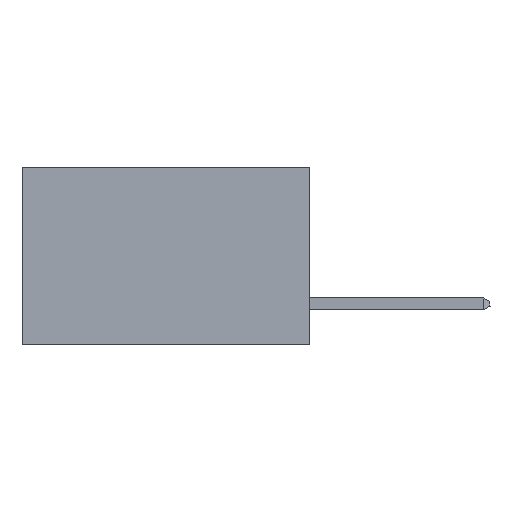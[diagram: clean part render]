
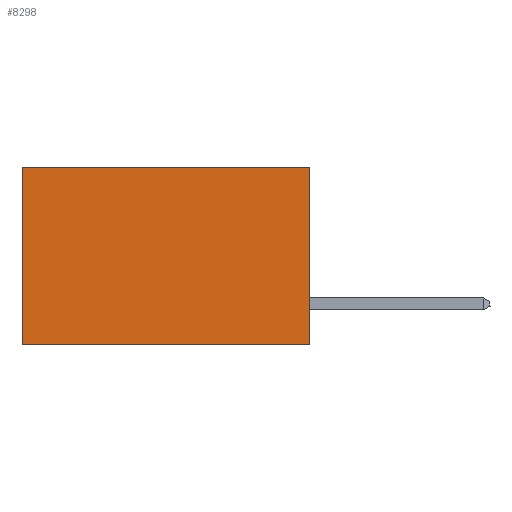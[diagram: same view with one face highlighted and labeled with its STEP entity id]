
A CAD part, left-side view. The second image highlights one B-rep face of the part: STEP entity #8298.
In plain terms, the highlighted planar face has unit normal (-1, 0, 0).
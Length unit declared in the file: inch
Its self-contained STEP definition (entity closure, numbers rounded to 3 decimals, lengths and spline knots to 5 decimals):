
#2330 = EDGE_CURVE ( 'NONE', #5590, #45355, #39319, .T. ) ;
#2902 = VECTOR ( 'NONE', #12301, 39.37008 ) ;
#4670 = CARTESIAN_POINT ( 'NONE',  ( 0.2875, 0., 0. ) ) ;
#5590 = VERTEX_POINT ( 'NONE', #4670 ) ;
#5637 = EDGE_CURVE ( 'NONE', #5590, #42489, #44893, .T. ) ;
#8045 = ORIENTED_EDGE ( 'NONE', *, *, #22477, .T. ) ;
#8128 = CARTESIAN_POINT ( 'NONE',  ( 0.2875, 0.6, 0. ) ) ;
#8298 = ADVANCED_FACE ( 'NONE', ( #40250 ), #26927, .F. ) ;
#8915 = LINE ( 'NONE', #32776, #2902 ) ;
#9253 = DIRECTION ( 'NONE',  ( 0., 0., -1. ) ) ;
#12110 = VECTOR ( 'NONE', #12383, 39.37008 ) ;
#12301 = DIRECTION ( 'NONE',  ( 0., 1., 0. ) ) ;
#12383 = DIRECTION ( 'NONE',  ( 0., 0., -1. ) ) ;
#12662 = CARTESIAN_POINT ( 'NONE',  ( 0.2875, 0., 0. ) ) ;
#14889 = CARTESIAN_POINT ( 'NONE',  ( 0.2875, 0.6, -0.37 ) ) ;
#21448 = LINE ( 'NONE', #8128, #12110 ) ;
#22477 = EDGE_CURVE ( 'NONE', #42489, #28965, #21448, .T. ) ;
#24565 = CARTESIAN_POINT ( 'NONE',  ( 0.2875, 0., 0. ) ) ;
#25160 = EDGE_LOOP ( 'NONE', ( #8045, #36801, #32295, #39297 ) ) ;
#25225 = CARTESIAN_POINT ( 'NONE',  ( 0.2875, 0., -0.37 ) ) ;
#26927 = PLANE ( 'NONE',  #27467 ) ;
#27467 = AXIS2_PLACEMENT_3D ( 'NONE', #37760, #40840, #9253 ) ;
#28876 = VECTOR ( 'NONE', #35573, 39.37008 ) ;
#28965 = VERTEX_POINT ( 'NONE', #14889 ) ;
#29364 = EDGE_CURVE ( 'NONE', #45355, #28965, #8915, .T. ) ;
#32295 = ORIENTED_EDGE ( 'NONE', *, *, #2330, .F. ) ;
#32776 = CARTESIAN_POINT ( 'NONE',  ( 0.2875, 0., -0.37 ) ) ;
#34335 = CARTESIAN_POINT ( 'NONE',  ( 0.2875, 0.6, 0. ) ) ;
#35573 = DIRECTION ( 'NONE',  ( 0., 1., 0. ) ) ;
#36801 = ORIENTED_EDGE ( 'NONE', *, *, #29364, .F. ) ;
#37760 = CARTESIAN_POINT ( 'NONE',  ( 0.2875, 0., 0. ) ) ;
#39297 = ORIENTED_EDGE ( 'NONE', *, *, #5637, .T. ) ;
#39319 = LINE ( 'NONE', #12662, #40425 ) ;
#40250 = FACE_OUTER_BOUND ( 'NONE', #25160, .T. ) ;
#40425 = VECTOR ( 'NONE', #41012, 39.37008 ) ;
#40840 = DIRECTION ( 'NONE',  ( 1., 0., 0. ) ) ;
#41012 = DIRECTION ( 'NONE',  ( 0., 0., -1. ) ) ;
#42489 = VERTEX_POINT ( 'NONE', #34335 ) ;
#44893 = LINE ( 'NONE', #24565, #28876 ) ;
#45355 = VERTEX_POINT ( 'NONE', #25225 ) ;
